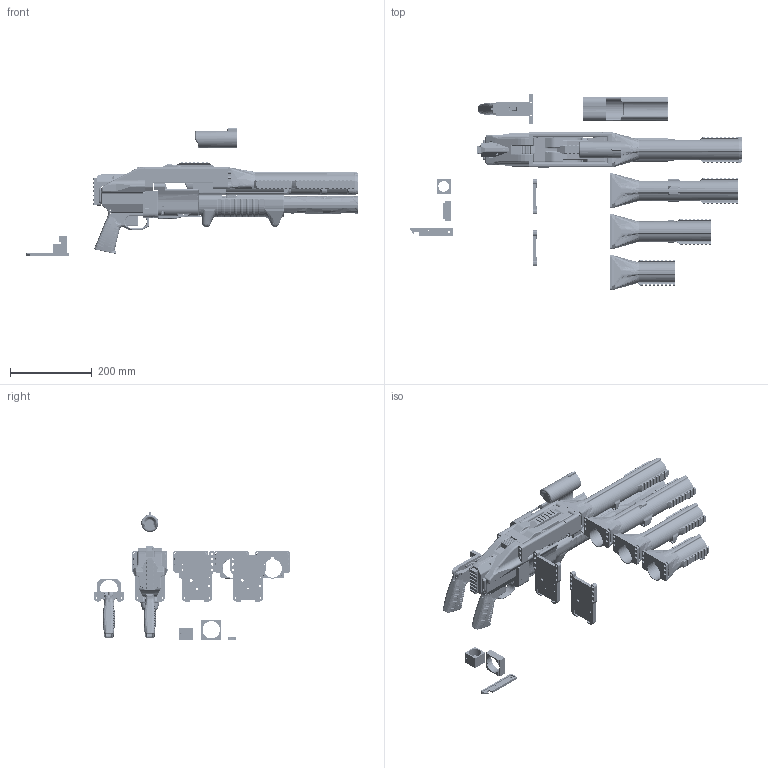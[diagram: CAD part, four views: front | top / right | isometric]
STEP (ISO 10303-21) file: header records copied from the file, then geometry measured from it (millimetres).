
FILE_DESCRIPTION(/* description */ (''),/* implementation_level */ '2;1');
FILE_NAME(/* name */ 'B.A.L.L.S. .step',/* time_stamp */ '2022-10-13T19:43:38-04:00',/* author */ (''),/* organization */ (''),/* preprocessor_version */ 'ST-DEVELOPER v19',/* originating_system */ 'Autodesk Translation Framework v11.7.0.108',/* authorisation */ '');
FILE_SCHEMA (('AUTOMOTIVE_DESIGN { 1 0 10303 214 3 1 1 }'));
Products named in the file (63): (Unsaved); A. Upper Assembly; A01. Magazine (Full-sized); A01.1. Magazine (Short); A01.2. Magazine (Medium); A01.3. Magazine (2-Peice Front); A01.3a. Magazine (2-Peice Rear); A01a. Magazine Cap; A01b. Follower; A01c. Follower (XL); A02. Trunion; A02a. Left Pannel; A02a. Right Pannel; A02b. Round Catch; A03. Lid; A03a. Pusher; A99. Spring Bending Jig; B. Lower Assembly; B00. Barrel; B00. Locking Arm (1); B00. Locking Arm; B00. Pump Guide ; B00. Pump Guide (1); B01. Barrel Retainer; B02. Pump (Type 1); B02.1. Pump (Type 2) (Beefy); B02a. Pump Button; B02b. Pump Collar (Top); B02c. Pump Collar (Bottom); B02d. Unlock Cam; B03. Locking Arm Connector; B99. Locking Tab Cut Cuide; B99. Chamber Cut Guide; C. Breech Assembly; C00. Rim Rail; C00. Rim Rail 2; C00. Locking Bar; C00. Breach Bar 1; C00. Breach Bar 2; C00. Breech Face  ...
Assembly tree (62 placements, depth 3):
  (Unsaved)
    A. Upper Assembly
      A01. Magazine (Full-sized)
      A01.1. Magazine (Short)
      A01.2. Magazine (Medium)
      A01.3. Magazine (2-Peice Front)
      A01.3a. Magazine (2-Peice Rear)
      A01a. Magazine Cap
      A01b. Follower
      A01c. Follower (XL)
      A02. Trunion
      A02a. Left Pannel
      A02a. Right Pannel
      A02b. Round Catch
      A03. Lid
      A03a. Pusher
      A99. Spring Bending Jig
    B. Lower Assembly
      B00. Barrel
      B00. Locking Arm (1)
      B00. Locking Arm
      B00. Pump Guide 
      B00. Pump Guide (1)
      B01. Barrel Retainer
      B02. Pump (Type 1)
      B02.1. Pump (Type 2) (Beefy)
      B02a. Pump Button
      B02b. Pump Collar (Top)
      B02c. Pump Collar (Bottom)
      B02d. Unlock Cam
      B03. Locking Arm Connector
      B99. Locking Tab Cut Cuide
      B99. Chamber Cut Guide
    C. Breech Assembly
      C00. Rim Rail
      C00. Rim Rail 2
      C00. Locking Bar
      C00. Breach Bar 1
      C00. Breach Bar 2
      C00. Breech Face 
      C01. Breach Plate (Reenforced)
      C01.1. Breach Plate (Printed)
      C01.2. Breach Plate (SCS Plate 3mm)
      C01a. Detent
      C03. Rim Plate (Right)
      C02. Rim Plate (Left)
    D. Receiver Assembly
      D00. Push Back Pin
      D00. Firing Pin
      D00. Striker Rod
      D00. Trigger Rod (1)
      D00. Trigger Rod
      D01. Receiver  Top
      D01a. Lid Catch
      D02. Receiver Cover (1)
      D03. Receiver Bottom (1 Spring)
      D03.1. Receiver Bottom (2 Spring)
      D03a. Sear Trip
      D04. Trigger (1 Spring)
      D04.1. Trigger (2 Spring)
Bounding box: 811.23 x 479.99 x 311.5 mm (x, y, z)
Volume: 3332037 mm3; surface area: 1274710.7 mm2
Topology: 58 solids, 58 shells, 6118 faces, 16177 edges, 10265 vertices
Faces by surface type: plane 2726, cylinder 1799, bspline 1038, torus 277, sphere 192, cone 86
Full cylindrical faces by diameter (mm): 2 x6, 2.15 x3, 2.5 x2, 3 x26, 3.1 x9, 3.2 x2, 3.25 x6, 3.3 x33, 3.4 x76, 3.5 x9, 4 x5, 4.4 x58, 5 x9, 5.25 x1, 5.422 x1, 5.423 x1, 5.5 x14, 6 x17, 6.1 x1, 6.2 x3, 6.25 x10, 6.3 x11, 6.5 x68, 7 x1, 8 x2, 12.25 x2, 26 x1, 30 x1, 37 x1, 39 x1
Entity records: 220419 total; most frequent: CARTESIAN_POINT 72638, ORIENTED_EDGE 32260, DIRECTION 28329, EDGE_CURVE 16130, VERTEX_POINT 10265, AXIS2_PLACEMENT_3D 9880, LINE 8569, VECTOR 8569
